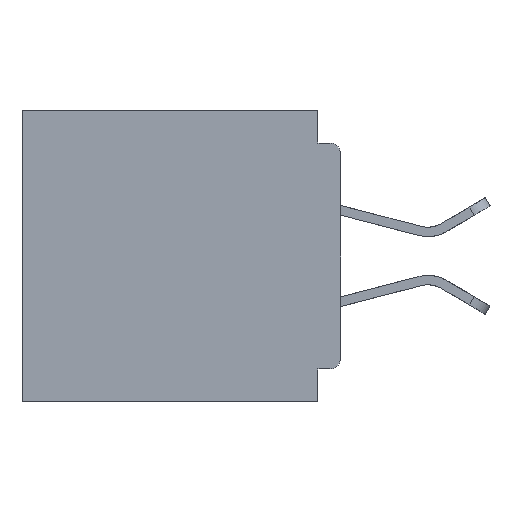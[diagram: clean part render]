
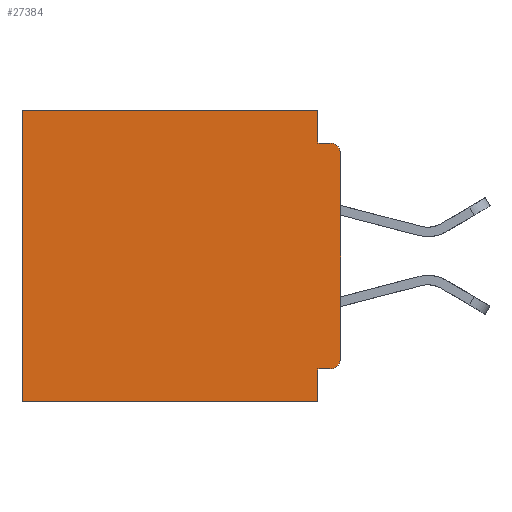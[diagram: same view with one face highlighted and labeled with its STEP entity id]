
A CAD part, left-side view. The second image highlights one B-rep face of the part: STEP entity #27384.
In plain terms, the highlighted planar face has unit normal (-1, 0, 0).
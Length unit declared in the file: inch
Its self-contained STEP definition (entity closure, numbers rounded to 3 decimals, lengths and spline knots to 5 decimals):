
#4 = VECTOR ( 'NONE', #16090, 39.37008 ) ;
#714 = LINE ( 'NONE', #10380, #33663 ) ;
#2913 = PLANE ( 'NONE',  #32004 ) ;
#3660 = LINE ( 'NONE', #37429, #28193 ) ;
#4005 = CARTESIAN_POINT ( 'NONE',  ( 0.3, 0.015, -0.34 ) ) ;
#4013 = VERTEX_POINT ( 'NONE', #33583 ) ;
#4574 = CARTESIAN_POINT ( 'NONE',  ( 0.3, 0.015, -0.045 ) ) ;
#4617 = CARTESIAN_POINT ( 'NONE',  ( 0.3, 0., 0. ) ) ;
#4838 = LINE ( 'NONE', #4617, #19829 ) ;
#5050 = CIRCLE ( 'NONE', #20871, 0.015 ) ;
#5399 = LINE ( 'NONE', #6759, #21431 ) ;
#6093 = DIRECTION ( 'NONE',  ( 0., 0., -1. ) ) ;
#6759 = CARTESIAN_POINT ( 'NONE',  ( 0.3, 0.031, -0.4 ) ) ;
#6995 = CIRCLE ( 'NONE', #18195, 0.015 ) ;
#7222 = DIRECTION ( 'NONE',  ( 0., 0., -1. ) ) ;
#8217 = LINE ( 'NONE', #32373, #16725 ) ;
#8360 = VECTOR ( 'NONE', #33479, 39.37008 ) ;
#9250 = EDGE_CURVE ( 'NONE', #19293, #40200, #5050, .T. ) ;
#10380 = CARTESIAN_POINT ( 'NONE',  ( 0.3, 0., -0.355 ) ) ;
#10762 = ORIENTED_EDGE ( 'NONE', *, *, #27115, .T. ) ;
#11165 = CARTESIAN_POINT ( 'NONE',  ( 0.3, 0.437, -0.4 ) ) ;
#12867 = CARTESIAN_POINT ( 'NONE',  ( 0.3, 0., -0.045 ) ) ;
#13034 = EDGE_CURVE ( 'NONE', #37631, #35475, #33931, .T. ) ;
#13297 = DIRECTION ( 'NONE',  ( 0., 1., 0. ) ) ;
#13803 = CARTESIAN_POINT ( 'NONE',  ( 0.3, 0.437, -0.4 ) ) ;
#14368 = EDGE_LOOP ( 'NONE', ( #38358, #22183, #30426, #38774, #31478, #10762, #23634, #37985, #41238, #31709 ) ) ;
#16090 = DIRECTION ( 'NONE',  ( 0., -1., 0. ) ) ;
#16725 = VECTOR ( 'NONE', #13297, 39.37008 ) ;
#17174 = VECTOR ( 'NONE', #20829, 39.37008 ) ;
#17566 = VERTEX_POINT ( 'NONE', #26654 ) ;
#17656 = CARTESIAN_POINT ( 'NONE',  ( 0.3, 0.015, -0.06 ) ) ;
#18195 = AXIS2_PLACEMENT_3D ( 'NONE', #17656, #39960, #20870 ) ;
#18880 = VERTEX_POINT ( 'NONE', #27405 ) ;
#19293 = VERTEX_POINT ( 'NONE', #38731 ) ;
#19829 = VECTOR ( 'NONE', #30054, 39.37008 ) ;
#20356 = CARTESIAN_POINT ( 'NONE',  ( 0.3, 0., -0.34 ) ) ;
#20829 = DIRECTION ( 'NONE',  ( 0., 0., -1. ) ) ;
#20870 = DIRECTION ( 'NONE',  ( 0., 0., -1. ) ) ;
#20871 = AXIS2_PLACEMENT_3D ( 'NONE', #4005, #26405, #7222 ) ;
#21346 = VERTEX_POINT ( 'NONE', #26914 ) ;
#21404 = EDGE_CURVE ( 'NONE', #21346, #35475, #6995, .T. ) ;
#21431 = VECTOR ( 'NONE', #35548, 39.37008 ) ;
#22055 = CARTESIAN_POINT ( 'NONE',  ( 0.3, 0., -0.4 ) ) ;
#22183 = ORIENTED_EDGE ( 'NONE', *, *, #21404, .T. ) ;
#22848 = FACE_OUTER_BOUND ( 'NONE', #14368, .T. ) ;
#23634 = ORIENTED_EDGE ( 'NONE', *, *, #30709, .F. ) ;
#25329 = DIRECTION ( 'NONE',  ( 1., 0., 0. ) ) ;
#25726 = LINE ( 'NONE', #39921, #17174 ) ;
#26405 = DIRECTION ( 'NONE',  ( -1., 0., 0. ) ) ;
#26654 = CARTESIAN_POINT ( 'NONE',  ( 0.3, 0.031, -0.355 ) ) ;
#26914 = CARTESIAN_POINT ( 'NONE',  ( 0.3, 0., -0.06 ) ) ;
#27115 = EDGE_CURVE ( 'NONE', #18880, #31342, #40304, .T. ) ;
#27384 = ADVANCED_FACE ( 'NONE', ( #22848 ), #2913, .F. ) ;
#27405 = CARTESIAN_POINT ( 'NONE',  ( 0.3, 0.437, 0. ) ) ;
#28193 = VECTOR ( 'NONE', #40626, 39.37008 ) ;
#30054 = DIRECTION ( 'NONE',  ( 0., 1., 0. ) ) ;
#30426 = ORIENTED_EDGE ( 'NONE', *, *, #13034, .F. ) ;
#30709 = EDGE_CURVE ( 'NONE', #35565, #31342, #8217, .T. ) ;
#31342 = VERTEX_POINT ( 'NONE', #13803 ) ;
#31478 = ORIENTED_EDGE ( 'NONE', *, *, #37616, .T. ) ;
#31709 = ORIENTED_EDGE ( 'NONE', *, *, #9250, .T. ) ;
#32004 = AXIS2_PLACEMENT_3D ( 'NONE', #22055, #25329, #6093 ) ;
#32373 = CARTESIAN_POINT ( 'NONE',  ( 0.3, 0., -0.4 ) ) ;
#32686 = DIRECTION ( 'NONE',  ( 0., 1., 0. ) ) ;
#33479 = DIRECTION ( 'NONE',  ( 0., 0., -1. ) ) ;
#33583 = CARTESIAN_POINT ( 'NONE',  ( 0.3, 0.031, 0. ) ) ;
#33663 = VECTOR ( 'NONE', #32686, 39.37008 ) ;
#33931 = LINE ( 'NONE', #12867, #4 ) ;
#35475 = VERTEX_POINT ( 'NONE', #4574 ) ;
#35548 = DIRECTION ( 'NONE',  ( 0., 0., -1. ) ) ;
#35565 = VERTEX_POINT ( 'NONE', #40034 ) ;
#36595 = CARTESIAN_POINT ( 'NONE',  ( 0.3, 0.031, -0.045 ) ) ;
#36916 = EDGE_CURVE ( 'NONE', #17566, #35565, #5399, .T. ) ;
#37429 = CARTESIAN_POINT ( 'NONE',  ( 0.3, 0.031, 0. ) ) ;
#37616 = EDGE_CURVE ( 'NONE', #4013, #18880, #4838, .T. ) ;
#37631 = VERTEX_POINT ( 'NONE', #36595 ) ;
#37985 = ORIENTED_EDGE ( 'NONE', *, *, #36916, .F. ) ;
#38358 = ORIENTED_EDGE ( 'NONE', *, *, #39591, .F. ) ;
#38731 = CARTESIAN_POINT ( 'NONE',  ( 0.3, 0.015, -0.355 ) ) ;
#38774 = ORIENTED_EDGE ( 'NONE', *, *, #39769, .F. ) ;
#39383 = EDGE_CURVE ( 'NONE', #19293, #17566, #714, .T. ) ;
#39591 = EDGE_CURVE ( 'NONE', #21346, #40200, #25726, .T. ) ;
#39769 = EDGE_CURVE ( 'NONE', #4013, #37631, #3660, .T. ) ;
#39921 = CARTESIAN_POINT ( 'NONE',  ( 0.3, 0., -0.4 ) ) ;
#39960 = DIRECTION ( 'NONE',  ( -1., 0., 0. ) ) ;
#40034 = CARTESIAN_POINT ( 'NONE',  ( 0.3, 0.031, -0.4 ) ) ;
#40200 = VERTEX_POINT ( 'NONE', #20356 ) ;
#40304 = LINE ( 'NONE', #11165, #8360 ) ;
#40626 = DIRECTION ( 'NONE',  ( 0., 0., -1. ) ) ;
#41238 = ORIENTED_EDGE ( 'NONE', *, *, #39383, .F. ) ;
